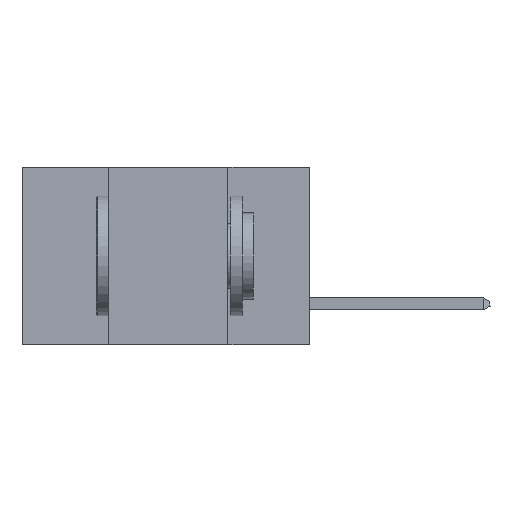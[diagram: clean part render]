
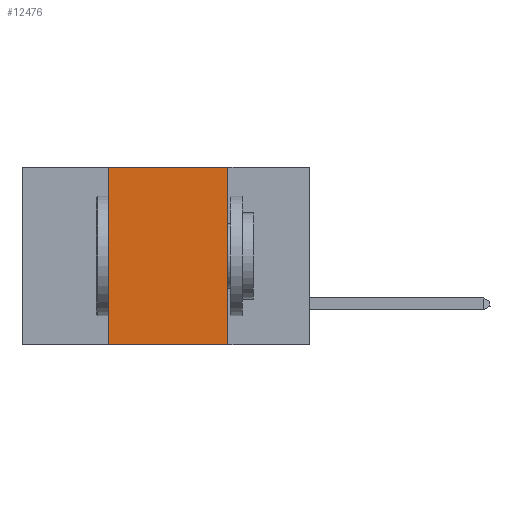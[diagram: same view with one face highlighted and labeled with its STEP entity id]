
A CAD part, left-side view. The second image highlights one B-rep face of the part: STEP entity #12476.
In plain terms, the highlighted planar face has unit normal (-1, 0, 0).
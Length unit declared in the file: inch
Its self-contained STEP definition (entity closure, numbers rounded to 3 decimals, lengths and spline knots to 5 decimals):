
#273 = ORIENTED_EDGE ( 'NONE', *, *, #5573, .F. ) ;
#438 = CARTESIAN_POINT ( 'NONE',  ( 0., 0.17, -0.37 ) ) ;
#470 = LINE ( 'NONE', #2756, #9384 ) ;
#826 = VECTOR ( 'NONE', #6125, 39.37008 ) ;
#849 = ORIENTED_EDGE ( 'NONE', *, *, #11937, .F. ) ;
#1146 = VECTOR ( 'NONE', #5782, 39.37008 ) ;
#1797 = EDGE_CURVE ( 'NONE', #11648, #10733, #11214, .T. ) ;
#2491 = VERTEX_POINT ( 'NONE', #438 ) ;
#2500 = CARTESIAN_POINT ( 'NONE',  ( 0., 0.42, -0.37 ) ) ;
#2756 = CARTESIAN_POINT ( 'NONE',  ( 0., 0.6, 0. ) ) ;
#2856 = AXIS2_PLACEMENT_3D ( 'NONE', #3448, #14024, #6953 ) ;
#3192 = LINE ( 'NONE', #10870, #826 ) ;
#3448 = CARTESIAN_POINT ( 'NONE',  ( 0., 0.6, 0. ) ) ;
#3972 = DIRECTION ( 'NONE',  ( 0., -1., 0. ) ) ;
#5573 = EDGE_CURVE ( 'NONE', #10733, #12406, #470, .T. ) ;
#5782 = DIRECTION ( 'NONE',  ( 0., 0., 1. ) ) ;
#6125 = DIRECTION ( 'NONE',  ( 0., 0., -1. ) ) ;
#6953 = DIRECTION ( 'NONE',  ( 0., 0., -1. ) ) ;
#6989 = LINE ( 'NONE', #14137, #11239 ) ;
#7076 = DIRECTION ( 'NONE',  ( 0., -1., 0. ) ) ;
#8136 = CARTESIAN_POINT ( 'NONE',  ( 0., 0.42, 0. ) ) ;
#8794 = FACE_OUTER_BOUND ( 'NONE', #12116, .T. ) ;
#8995 = CARTESIAN_POINT ( 'NONE',  ( 0., 0.17, 0. ) ) ;
#9235 = PLANE ( 'NONE',  #2856 ) ;
#9384 = VECTOR ( 'NONE', #3972, 39.37008 ) ;
#10733 = VERTEX_POINT ( 'NONE', #13064 ) ;
#10824 = ORIENTED_EDGE ( 'NONE', *, *, #12231, .T. ) ;
#10870 = CARTESIAN_POINT ( 'NONE',  ( 0., 0.17, 0. ) ) ;
#11214 = LINE ( 'NONE', #8136, #1146 ) ;
#11239 = VECTOR ( 'NONE', #7076, 39.37008 ) ;
#11648 = VERTEX_POINT ( 'NONE', #2500 ) ;
#11937 = EDGE_CURVE ( 'NONE', #12406, #2491, #3192, .T. ) ;
#12116 = EDGE_LOOP ( 'NONE', ( #849, #273, #13092, #10824 ) ) ;
#12231 = EDGE_CURVE ( 'NONE', #11648, #2491, #6989, .T. ) ;
#12406 = VERTEX_POINT ( 'NONE', #8995 ) ;
#12476 = ADVANCED_FACE ( 'NONE', ( #8794 ), #9235, .F. ) ;
#13064 = CARTESIAN_POINT ( 'NONE',  ( 0., 0.42, 0. ) ) ;
#13092 = ORIENTED_EDGE ( 'NONE', *, *, #1797, .F. ) ;
#14024 = DIRECTION ( 'NONE',  ( 1., 0., 0. ) ) ;
#14137 = CARTESIAN_POINT ( 'NONE',  ( 0., 0.6, -0.37 ) ) ;
